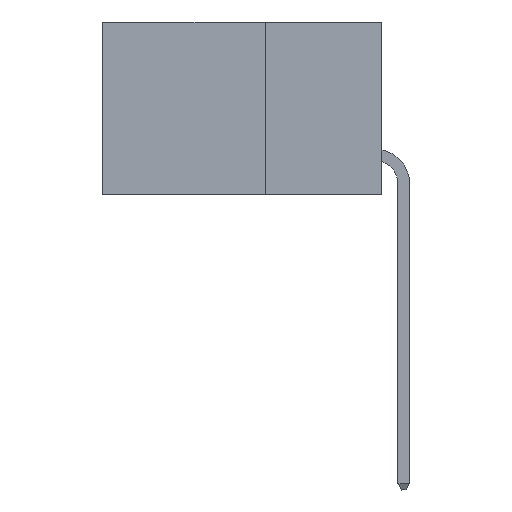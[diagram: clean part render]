
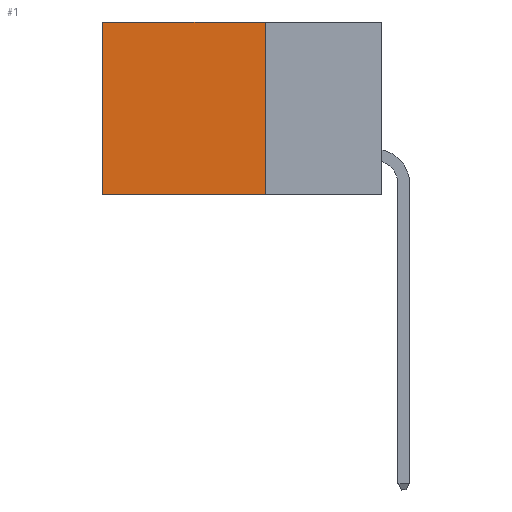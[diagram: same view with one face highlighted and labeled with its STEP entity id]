
A CAD part, left-side view. The second image highlights one B-rep face of the part: STEP entity #1.
In plain terms, the highlighted planar face has unit normal (-1, 0, 0).
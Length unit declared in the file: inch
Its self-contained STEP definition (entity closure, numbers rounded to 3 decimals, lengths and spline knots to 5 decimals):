
#1 = ADVANCED_FACE ( 'NONE', ( #6669 ), #1444, .F. ) ;
#351 = VERTEX_POINT ( 'NONE', #9052 ) ;
#376 = LINE ( 'NONE', #2906, #5740 ) ;
#1262 = EDGE_CURVE ( 'NONE', #4665, #1709, #9077, .T. ) ;
#1444 = PLANE ( 'NONE',  #9116 ) ;
#1709 = VERTEX_POINT ( 'NONE', #11498 ) ;
#2248 = CARTESIAN_POINT ( 'NONE',  ( 0.2875, 0.25, 0. ) ) ;
#2906 = CARTESIAN_POINT ( 'NONE',  ( 0.2875, 0.6, 0. ) ) ;
#3043 = EDGE_CURVE ( 'NONE', #4665, #351, #8428, .T. ) ;
#3366 = DIRECTION ( 'NONE',  ( 0., 1., 0. ) ) ;
#3382 = CARTESIAN_POINT ( 'NONE',  ( 0.2875, 0.6, -0.37 ) ) ;
#3906 = DIRECTION ( 'NONE',  ( 0., 0., -1. ) ) ;
#4582 = DIRECTION ( 'NONE',  ( 1., 0., 0. ) ) ;
#4665 = VERTEX_POINT ( 'NONE', #7007 ) ;
#5614 = VECTOR ( 'NONE', #3906, 39.37008 ) ;
#5646 = CARTESIAN_POINT ( 'NONE',  ( 0.2875, 0.25, 0. ) ) ;
#5740 = VECTOR ( 'NONE', #11816, 39.37008 ) ;
#6039 = ORIENTED_EDGE ( 'NONE', *, *, #9438, .T. ) ;
#6669 = FACE_OUTER_BOUND ( 'NONE', #6849, .T. ) ;
#6849 = EDGE_LOOP ( 'NONE', ( #6039, #7819, #10434, #14197 ) ) ;
#7007 = CARTESIAN_POINT ( 'NONE',  ( 0.2875, 0.25, 0. ) ) ;
#7819 = ORIENTED_EDGE ( 'NONE', *, *, #13653, .F. ) ;
#8428 = LINE ( 'NONE', #2248, #13158 ) ;
#9052 = CARTESIAN_POINT ( 'NONE',  ( 0.2875, 0.6, 0. ) ) ;
#9077 = LINE ( 'NONE', #12706, #5614 ) ;
#9085 = LINE ( 'NONE', #11467, #9956 ) ;
#9116 = AXIS2_PLACEMENT_3D ( 'NONE', #5646, #4582, #12360 ) ;
#9438 = EDGE_CURVE ( 'NONE', #351, #10035, #376, .T. ) ;
#9956 = VECTOR ( 'NONE', #13626, 39.37008 ) ;
#10035 = VERTEX_POINT ( 'NONE', #3382 ) ;
#10434 = ORIENTED_EDGE ( 'NONE', *, *, #1262, .F. ) ;
#11467 = CARTESIAN_POINT ( 'NONE',  ( 0.2875, 0.25, -0.37 ) ) ;
#11498 = CARTESIAN_POINT ( 'NONE',  ( 0.2875, 0.25, -0.37 ) ) ;
#11816 = DIRECTION ( 'NONE',  ( 0., 0., -1. ) ) ;
#12360 = DIRECTION ( 'NONE',  ( 0., 0., -1. ) ) ;
#12706 = CARTESIAN_POINT ( 'NONE',  ( 0.2875, 0.25, 0. ) ) ;
#13158 = VECTOR ( 'NONE', #3366, 39.37008 ) ;
#13626 = DIRECTION ( 'NONE',  ( 0., 1., 0. ) ) ;
#13653 = EDGE_CURVE ( 'NONE', #1709, #10035, #9085, .T. ) ;
#14197 = ORIENTED_EDGE ( 'NONE', *, *, #3043, .T. ) ;
